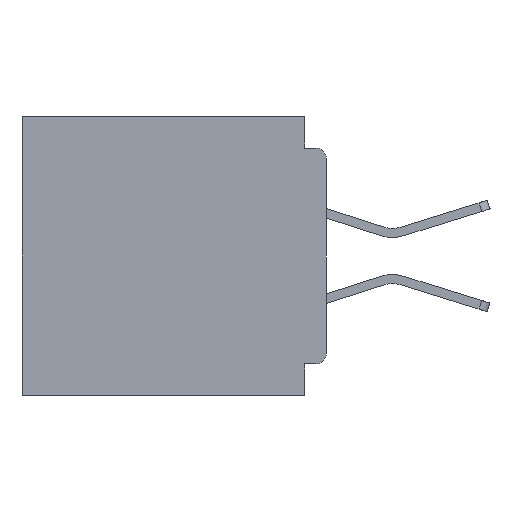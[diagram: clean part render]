
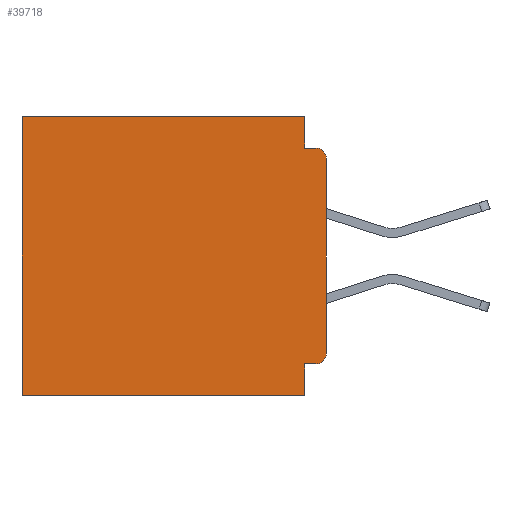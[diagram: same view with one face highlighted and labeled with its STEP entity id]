
A CAD part, left-side view. The second image highlights one B-rep face of the part: STEP entity #39718.
In plain terms, the highlighted planar face has unit normal (-1, 0, 0).
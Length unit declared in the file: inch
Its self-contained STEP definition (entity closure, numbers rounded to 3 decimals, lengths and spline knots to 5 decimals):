
#383 = DIRECTION ( 'NONE',  ( 0., 1., 0. ) ) ;
#786 = EDGE_CURVE ( 'NONE', #45329, #22687, #24360, .T. ) ;
#1318 = LINE ( 'NONE', #38664, #32529 ) ;
#2842 = CARTESIAN_POINT ( 'NONE',  ( 0.3, 0.031, -0.4 ) ) ;
#4042 = DIRECTION ( 'NONE',  ( 0., 1., 0. ) ) ;
#4473 = CARTESIAN_POINT ( 'NONE',  ( 0.3, 0.015, -0.355 ) ) ;
#4791 = ORIENTED_EDGE ( 'NONE', *, *, #10063, .F. ) ;
#5469 = CARTESIAN_POINT ( 'NONE',  ( 0.3, 0., -0.06 ) ) ;
#5502 = VERTEX_POINT ( 'NONE', #2842 ) ;
#5773 = VECTOR ( 'NONE', #26601, 39.37008 ) ;
#5847 = DIRECTION ( 'NONE',  ( -1., 0., 0. ) ) ;
#5963 = VERTEX_POINT ( 'NONE', #44204 ) ;
#6405 = VECTOR ( 'NONE', #4042, 39.37008 ) ;
#6636 = CARTESIAN_POINT ( 'NONE',  ( 0.3, 0., 0. ) ) ;
#6721 = EDGE_CURVE ( 'NONE', #5963, #29401, #14972, .T. ) ;
#7392 = ORIENTED_EDGE ( 'NONE', *, *, #17880, .F. ) ;
#8094 = CARTESIAN_POINT ( 'NONE',  ( 0.3, 0., -0.4 ) ) ;
#8181 = VERTEX_POINT ( 'NONE', #27195 ) ;
#9124 = AXIS2_PLACEMENT_3D ( 'NONE', #31240, #5847, #35571 ) ;
#9282 = CIRCLE ( 'NONE', #9124, 0.015 ) ;
#10063 = EDGE_CURVE ( 'NONE', #45329, #27410, #43801, .T. ) ;
#10213 = CARTESIAN_POINT ( 'NONE',  ( 0.3, 0.031, 0. ) ) ;
#10425 = EDGE_LOOP ( 'NONE', ( #4791, #25969, #20405, #33200, #44678, #19128, #29096, #13177, #7392, #53890 ) ) ;
#11524 = EDGE_CURVE ( 'NONE', #29401, #39821, #17082, .T. ) ;
#12335 = LINE ( 'NONE', #10213, #44856 ) ;
#12374 = DIRECTION ( 'NONE',  ( 1., 0., 0. ) ) ;
#12597 = VERTEX_POINT ( 'NONE', #4473 ) ;
#12641 = CARTESIAN_POINT ( 'NONE',  ( 0.3, 0., -0.34 ) ) ;
#13177 = ORIENTED_EDGE ( 'NONE', *, *, #42346, .F. ) ;
#14623 = DIRECTION ( 'NONE',  ( 0., 0., -1. ) ) ;
#14972 = LINE ( 'NONE', #6636, #23527 ) ;
#16083 = EDGE_CURVE ( 'NONE', #12597, #27410, #9282, .T. ) ;
#17082 = LINE ( 'NONE', #52092, #5773 ) ;
#17491 = CARTESIAN_POINT ( 'NONE',  ( 0.3, 0.031, -0.045 ) ) ;
#17812 = AXIS2_PLACEMENT_3D ( 'NONE', #54528, #42846, #48131 ) ;
#17880 = EDGE_CURVE ( 'NONE', #12597, #8181, #40297, .T. ) ;
#18133 = CARTESIAN_POINT ( 'NONE',  ( 0.3, 0.031, -0.4 ) ) ;
#18888 = CARTESIAN_POINT ( 'NONE',  ( 0.3, 0., -0.4 ) ) ;
#19128 = ORIENTED_EDGE ( 'NONE', *, *, #11524, .T. ) ;
#20157 = CARTESIAN_POINT ( 'NONE',  ( 0.3, 0., -0.045 ) ) ;
#20405 = ORIENTED_EDGE ( 'NONE', *, *, #22461, .F. ) ;
#21178 = VECTOR ( 'NONE', #14623, 39.37008 ) ;
#21590 = FACE_OUTER_BOUND ( 'NONE', #10425, .T. ) ;
#22461 = EDGE_CURVE ( 'NONE', #31749, #22687, #46917, .T. ) ;
#22687 = VERTEX_POINT ( 'NONE', #34473 ) ;
#23527 = VECTOR ( 'NONE', #27722, 39.37008 ) ;
#24352 = DIRECTION ( 'NONE',  ( 0., -1., 0. ) ) ;
#24360 = CIRCLE ( 'NONE', #17812, 0.015 ) ;
#25529 = EDGE_CURVE ( 'NONE', #5502, #39821, #1318, .T. ) ;
#25636 = CARTESIAN_POINT ( 'NONE',  ( 0.3, 0.437, -0.4 ) ) ;
#25969 = ORIENTED_EDGE ( 'NONE', *, *, #786, .T. ) ;
#25981 = VECTOR ( 'NONE', #47843, 39.37008 ) ;
#26601 = DIRECTION ( 'NONE',  ( 0., 0., -1. ) ) ;
#27195 = CARTESIAN_POINT ( 'NONE',  ( 0.3, 0.031, -0.355 ) ) ;
#27410 = VERTEX_POINT ( 'NONE', #12641 ) ;
#27722 = DIRECTION ( 'NONE',  ( 0., 1., 0. ) ) ;
#28287 = EDGE_CURVE ( 'NONE', #5963, #31749, #12335, .T. ) ;
#29096 = ORIENTED_EDGE ( 'NONE', *, *, #25529, .F. ) ;
#29401 = VERTEX_POINT ( 'NONE', #47433 ) ;
#31240 = CARTESIAN_POINT ( 'NONE',  ( 0.3, 0.015, -0.34 ) ) ;
#31749 = VERTEX_POINT ( 'NONE', #17491 ) ;
#32529 = VECTOR ( 'NONE', #383, 39.37008 ) ;
#33200 = ORIENTED_EDGE ( 'NONE', *, *, #28287, .F. ) ;
#33524 = PLANE ( 'NONE',  #41596 ) ;
#33764 = CARTESIAN_POINT ( 'NONE',  ( 0.3, 0., -0.355 ) ) ;
#34473 = CARTESIAN_POINT ( 'NONE',  ( 0.3, 0.015, -0.045 ) ) ;
#35571 = DIRECTION ( 'NONE',  ( 0., 0., -1. ) ) ;
#38664 = CARTESIAN_POINT ( 'NONE',  ( 0.3, 0., -0.4 ) ) ;
#39718 = ADVANCED_FACE ( 'NONE', ( #21590 ), #33524, .F. ) ;
#39821 = VERTEX_POINT ( 'NONE', #25636 ) ;
#40297 = LINE ( 'NONE', #33764, #6405 ) ;
#41596 = AXIS2_PLACEMENT_3D ( 'NONE', #8094, #12374, #42073 ) ;
#42073 = DIRECTION ( 'NONE',  ( 0., 0., -1. ) ) ;
#42346 = EDGE_CURVE ( 'NONE', #8181, #5502, #49979, .T. ) ;
#42846 = DIRECTION ( 'NONE',  ( -1., 0., 0. ) ) ;
#43801 = LINE ( 'NONE', #18888, #21178 ) ;
#44189 = DIRECTION ( 'NONE',  ( 0., 0., -1. ) ) ;
#44204 = CARTESIAN_POINT ( 'NONE',  ( 0.3, 0.031, 0. ) ) ;
#44234 = VECTOR ( 'NONE', #24352, 39.37008 ) ;
#44678 = ORIENTED_EDGE ( 'NONE', *, *, #6721, .T. ) ;
#44856 = VECTOR ( 'NONE', #44189, 39.37008 ) ;
#45329 = VERTEX_POINT ( 'NONE', #5469 ) ;
#46917 = LINE ( 'NONE', #20157, #44234 ) ;
#47433 = CARTESIAN_POINT ( 'NONE',  ( 0.3, 0.437, 0. ) ) ;
#47843 = DIRECTION ( 'NONE',  ( 0., 0., -1. ) ) ;
#48131 = DIRECTION ( 'NONE',  ( 0., 0., -1. ) ) ;
#49979 = LINE ( 'NONE', #18133, #25981 ) ;
#52092 = CARTESIAN_POINT ( 'NONE',  ( 0.3, 0.437, -0.4 ) ) ;
#53890 = ORIENTED_EDGE ( 'NONE', *, *, #16083, .T. ) ;
#54528 = CARTESIAN_POINT ( 'NONE',  ( 0.3, 0.015, -0.06 ) ) ;
